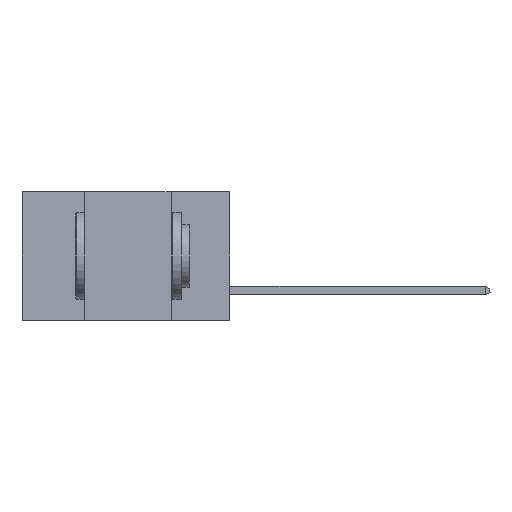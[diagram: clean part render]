
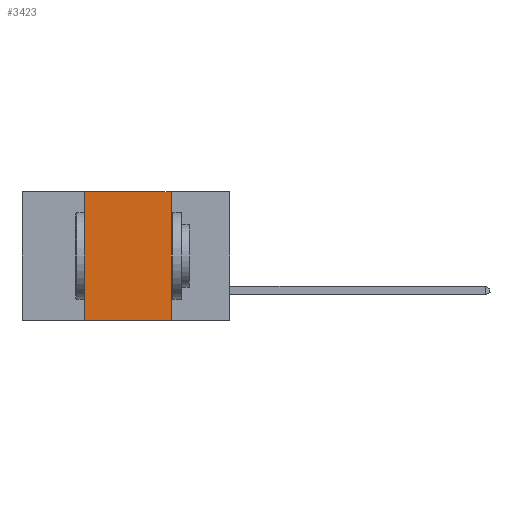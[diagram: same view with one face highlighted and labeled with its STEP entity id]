
A CAD part, left-side view. The second image highlights one B-rep face of the part: STEP entity #3423.
In plain terms, the highlighted planar face has unit normal (-1, 0, 0).
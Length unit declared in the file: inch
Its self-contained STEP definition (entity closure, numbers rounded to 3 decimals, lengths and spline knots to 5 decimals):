
#931 = ORIENTED_EDGE ( 'NONE', *, *, #3142, .F. ) ;
#2504 = EDGE_CURVE ( 'NONE', #6056, #17461, #8913, .T. ) ;
#2911 = LINE ( 'NONE', #6048, #13270 ) ;
#3142 = EDGE_CURVE ( 'NONE', #13091, #8132, #2911, .T. ) ;
#3423 = ADVANCED_FACE ( 'NONE', ( #16851 ), #13214, .F. ) ;
#3901 = CARTESIAN_POINT ( 'NONE',  ( 0., 0.17, 0. ) ) ;
#4166 = EDGE_CURVE ( 'NONE', #17461, #13091, #6507, .T. ) ;
#4516 = CARTESIAN_POINT ( 'NONE',  ( 0., 0.42, -0.37 ) ) ;
#4951 = CARTESIAN_POINT ( 'NONE',  ( 0., 0.6, 0. ) ) ;
#5209 = CARTESIAN_POINT ( 'NONE',  ( 0., 0.6, 0. ) ) ;
#6048 = CARTESIAN_POINT ( 'NONE',  ( 0., 0.17, 0. ) ) ;
#6056 = VERTEX_POINT ( 'NONE', #4516 ) ;
#6507 = LINE ( 'NONE', #5209, #18673 ) ;
#6717 = CARTESIAN_POINT ( 'NONE',  ( 0., 0.6, -0.37 ) ) ;
#7895 = ORIENTED_EDGE ( 'NONE', *, *, #4166, .F. ) ;
#8132 = VERTEX_POINT ( 'NONE', #13006 ) ;
#8442 = DIRECTION ( 'NONE',  ( 0., 0., -1. ) ) ;
#8842 = EDGE_LOOP ( 'NONE', ( #931, #7895, #14969, #14033 ) ) ;
#8913 = LINE ( 'NONE', #14198, #15109 ) ;
#9261 = DIRECTION ( 'NONE',  ( 0., 0., -1. ) ) ;
#10033 = DIRECTION ( 'NONE',  ( 1., 0., 0. ) ) ;
#12399 = VECTOR ( 'NONE', #14821, 39.37008 ) ;
#13006 = CARTESIAN_POINT ( 'NONE',  ( 0., 0.17, -0.37 ) ) ;
#13091 = VERTEX_POINT ( 'NONE', #3901 ) ;
#13188 = LINE ( 'NONE', #6717, #12399 ) ;
#13214 = PLANE ( 'NONE',  #15550 ) ;
#13268 = EDGE_CURVE ( 'NONE', #6056, #8132, #13188, .T. ) ;
#13270 = VECTOR ( 'NONE', #9261, 39.37008 ) ;
#13901 = CARTESIAN_POINT ( 'NONE',  ( 0., 0.42, 0. ) ) ;
#14033 = ORIENTED_EDGE ( 'NONE', *, *, #13268, .T. ) ;
#14198 = CARTESIAN_POINT ( 'NONE',  ( 0., 0.42, 0. ) ) ;
#14821 = DIRECTION ( 'NONE',  ( 0., -1., 0. ) ) ;
#14969 = ORIENTED_EDGE ( 'NONE', *, *, #2504, .F. ) ;
#15109 = VECTOR ( 'NONE', #15707, 39.37008 ) ;
#15205 = DIRECTION ( 'NONE',  ( 0., -1., 0. ) ) ;
#15550 = AXIS2_PLACEMENT_3D ( 'NONE', #4951, #10033, #8442 ) ;
#15707 = DIRECTION ( 'NONE',  ( 0., 0., 1. ) ) ;
#16851 = FACE_OUTER_BOUND ( 'NONE', #8842, .T. ) ;
#17461 = VERTEX_POINT ( 'NONE', #13901 ) ;
#18673 = VECTOR ( 'NONE', #15205, 39.37008 ) ;
